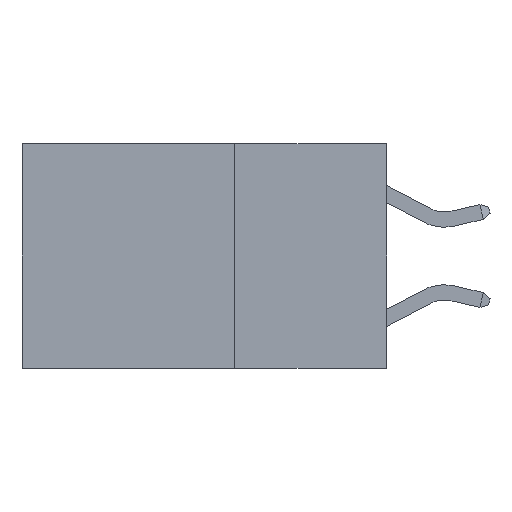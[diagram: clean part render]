
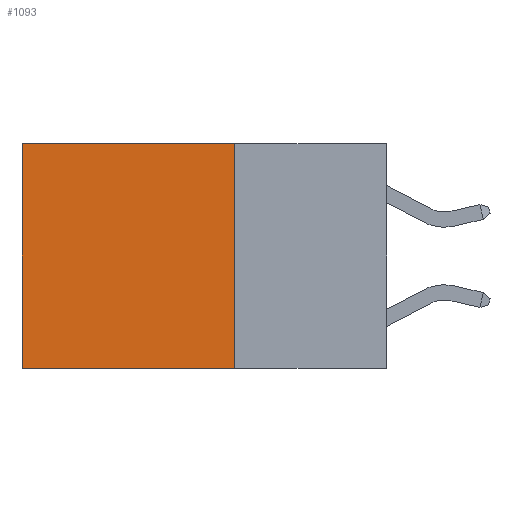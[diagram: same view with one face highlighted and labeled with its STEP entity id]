
A CAD part, left-side view. The second image highlights one B-rep face of the part: STEP entity #1093.
In plain terms, the highlighted planar face has unit normal (-1, 0, 0).
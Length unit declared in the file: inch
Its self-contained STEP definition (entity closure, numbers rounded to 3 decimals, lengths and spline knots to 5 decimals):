
#36 = ORIENTED_EDGE ( 'NONE', *, *, #4655, .F. ) ;
#524 = DIRECTION ( 'NONE',  ( 0., 1., 0. ) ) ;
#558 = EDGE_CURVE ( 'NONE', #8041, #1840, #2251, .T. ) ;
#656 = CARTESIAN_POINT ( 'NONE',  ( 0.2625, 0.25, 0. ) ) ;
#882 = EDGE_CURVE ( 'NONE', #2368, #11948, #3136, .T. ) ;
#1093 = ADVANCED_FACE ( 'NONE', ( #9358 ), #20509, .F. ) ;
#1840 = VERTEX_POINT ( 'NONE', #12478 ) ;
#2251 = LINE ( 'NONE', #656, #4390 ) ;
#2368 = VERTEX_POINT ( 'NONE', #9968 ) ;
#3136 = LINE ( 'NONE', #6608, #12390 ) ;
#4390 = VECTOR ( 'NONE', #16786, 39.37008 ) ;
#4655 = EDGE_CURVE ( 'NONE', #1840, #11948, #7147, .T. ) ;
#4811 = DIRECTION ( 'NONE',  ( 0., 0., -1. ) ) ;
#6371 = VECTOR ( 'NONE', #524, 39.37008 ) ;
#6608 = CARTESIAN_POINT ( 'NONE',  ( 0.2625, 0.6, 0. ) ) ;
#7147 = LINE ( 'NONE', #16737, #7871 ) ;
#7871 = VECTOR ( 'NONE', #13597, 39.37008 ) ;
#8041 = VERTEX_POINT ( 'NONE', #11469 ) ;
#9358 = FACE_OUTER_BOUND ( 'NONE', #16793, .T. ) ;
#9968 = CARTESIAN_POINT ( 'NONE',  ( 0.2625, 0.6, 0. ) ) ;
#11469 = CARTESIAN_POINT ( 'NONE',  ( 0.2625, 0.25, 0. ) ) ;
#11943 = CARTESIAN_POINT ( 'NONE',  ( 0.2625, 0.25, 0. ) ) ;
#11948 = VERTEX_POINT ( 'NONE', #17097 ) ;
#12020 = AXIS2_PLACEMENT_3D ( 'NONE', #17774, #20691, #4811 ) ;
#12390 = VECTOR ( 'NONE', #12963, 39.37008 ) ;
#12478 = CARTESIAN_POINT ( 'NONE',  ( 0.2625, 0.25, -0.37 ) ) ;
#12963 = DIRECTION ( 'NONE',  ( 0., 0., -1. ) ) ;
#13000 = EDGE_CURVE ( 'NONE', #8041, #2368, #15292, .T. ) ;
#13597 = DIRECTION ( 'NONE',  ( 0., 1., 0. ) ) ;
#15292 = LINE ( 'NONE', #11943, #6371 ) ;
#16737 = CARTESIAN_POINT ( 'NONE',  ( 0.2625, 0.25, -0.37 ) ) ;
#16786 = DIRECTION ( 'NONE',  ( 0., 0., -1. ) ) ;
#16793 = EDGE_LOOP ( 'NONE', ( #18912, #36, #17855, #20485 ) ) ;
#17097 = CARTESIAN_POINT ( 'NONE',  ( 0.2625, 0.6, -0.37 ) ) ;
#17774 = CARTESIAN_POINT ( 'NONE',  ( 0.2625, 0.25, 0. ) ) ;
#17855 = ORIENTED_EDGE ( 'NONE', *, *, #558, .F. ) ;
#18912 = ORIENTED_EDGE ( 'NONE', *, *, #882, .T. ) ;
#20485 = ORIENTED_EDGE ( 'NONE', *, *, #13000, .T. ) ;
#20509 = PLANE ( 'NONE',  #12020 ) ;
#20691 = DIRECTION ( 'NONE',  ( 1., 0., 0. ) ) ;
